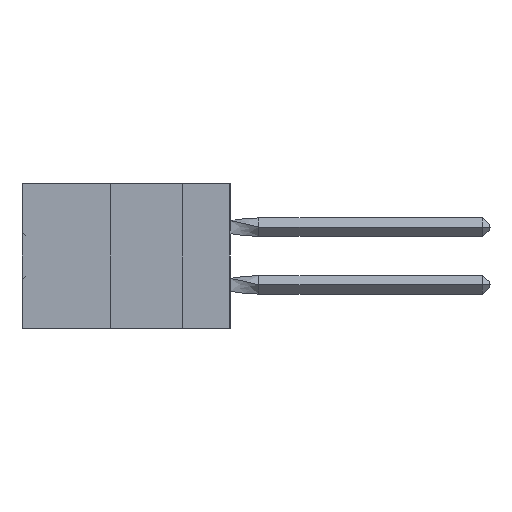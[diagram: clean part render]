
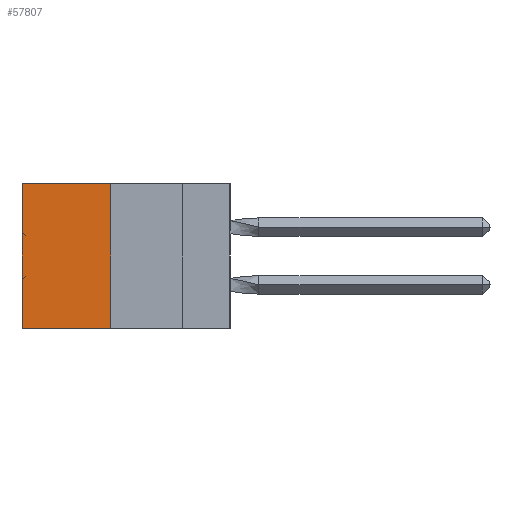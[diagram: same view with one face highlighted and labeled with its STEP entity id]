
A CAD part, left-side view. The second image highlights one B-rep face of the part: STEP entity #57807.
In plain terms, the highlighted planar face has unit normal (-1, 0, 0).
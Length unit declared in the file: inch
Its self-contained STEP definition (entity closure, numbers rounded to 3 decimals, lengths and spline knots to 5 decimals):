
#64 = EDGE_CURVE ( 'NONE', #17567, #43896, #53866, .T. ) ;
#1567 = DIRECTION ( 'NONE',  ( 0., 1., 0. ) ) ;
#3900 = LINE ( 'NONE', #48477, #57629 ) ;
#8874 = EDGE_CURVE ( 'NONE', #30526, #43896, #3900, .T. ) ;
#10249 = EDGE_CURVE ( 'NONE', #50092, #30526, #14511, .T. ) ;
#10616 = CARTESIAN_POINT ( 'NONE',  ( 0.305, 0.413, 0. ) ) ;
#11535 = ORIENTED_EDGE ( 'NONE', *, *, #64, .F. ) ;
#14511 = LINE ( 'NONE', #10616, #49563 ) ;
#14643 = FACE_OUTER_BOUND ( 'NONE', #18130, .T. ) ;
#15718 = DIRECTION ( 'NONE',  ( 1., 0., 0. ) ) ;
#17567 = VERTEX_POINT ( 'NONE', #55183 ) ;
#18130 = EDGE_LOOP ( 'NONE', ( #37869, #11535, #48147, #39286 ) ) ;
#24127 = CARTESIAN_POINT ( 'NONE',  ( 0.305, 0.413, -0.5 ) ) ;
#26607 = VECTOR ( 'NONE', #40348, 39.37008 ) ;
#27824 = CARTESIAN_POINT ( 'NONE',  ( 0.305, 0.72, -0.5 ) ) ;
#28415 = DIRECTION ( 'NONE',  ( 0., 0., -1. ) ) ;
#29750 = CARTESIAN_POINT ( 'NONE',  ( 0.305, 0.72, 0. ) ) ;
#30526 = VERTEX_POINT ( 'NONE', #29750 ) ;
#30764 = CARTESIAN_POINT ( 'NONE',  ( 0.305, 0.413, -0.5 ) ) ;
#30869 = VECTOR ( 'NONE', #28415, 39.37008 ) ;
#37869 = ORIENTED_EDGE ( 'NONE', *, *, #8874, .T. ) ;
#37983 = PLANE ( 'NONE',  #57468 ) ;
#38370 = DIRECTION ( 'NONE',  ( 0., 0., -1. ) ) ;
#39286 = ORIENTED_EDGE ( 'NONE', *, *, #10249, .T. ) ;
#40348 = DIRECTION ( 'NONE',  ( 0., 1., 0. ) ) ;
#41584 = LINE ( 'NONE', #50611, #30869 ) ;
#43896 = VERTEX_POINT ( 'NONE', #27824 ) ;
#48147 = ORIENTED_EDGE ( 'NONE', *, *, #53744, .F. ) ;
#48477 = CARTESIAN_POINT ( 'NONE',  ( 0.305, 0.72, -0.5 ) ) ;
#49563 = VECTOR ( 'NONE', #1567, 39.37008 ) ;
#50092 = VERTEX_POINT ( 'NONE', #55460 ) ;
#50611 = CARTESIAN_POINT ( 'NONE',  ( 0.305, 0.413, -0.5 ) ) ;
#53744 = EDGE_CURVE ( 'NONE', #50092, #17567, #41584, .T. ) ;
#53866 = LINE ( 'NONE', #30764, #26607 ) ;
#55183 = CARTESIAN_POINT ( 'NONE',  ( 0.305, 0.413, -0.5 ) ) ;
#55460 = CARTESIAN_POINT ( 'NONE',  ( 0.305, 0.413, 0. ) ) ;
#57089 = DIRECTION ( 'NONE',  ( 0., 0., -1. ) ) ;
#57468 = AXIS2_PLACEMENT_3D ( 'NONE', #24127, #15718, #38370 ) ;
#57629 = VECTOR ( 'NONE', #57089, 39.37008 ) ;
#57807 = ADVANCED_FACE ( 'NONE', ( #14643 ), #37983, .F. ) ;
